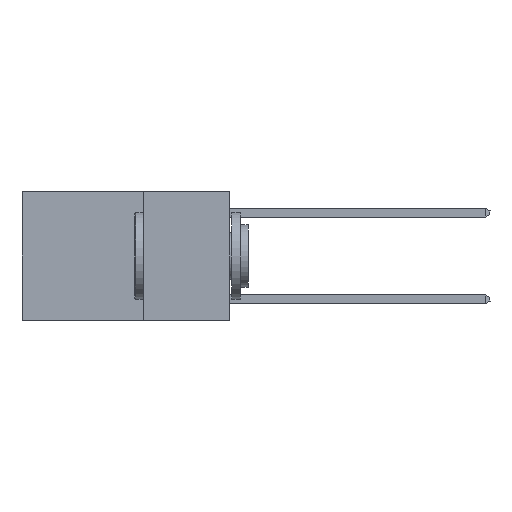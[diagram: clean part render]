
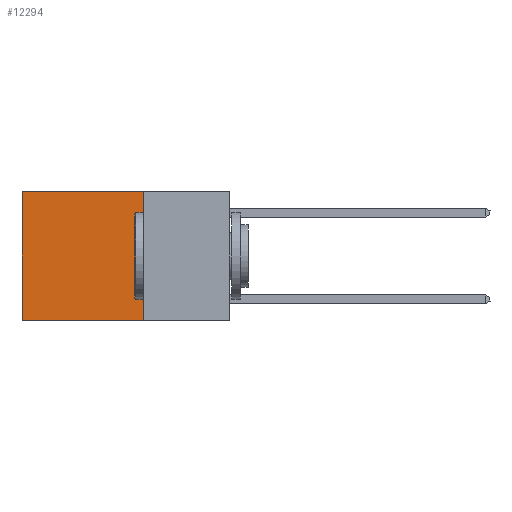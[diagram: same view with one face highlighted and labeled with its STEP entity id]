
A CAD part, left-side view. The second image highlights one B-rep face of the part: STEP entity #12294.
In plain terms, the highlighted planar face has unit normal (-1, 0, 0).
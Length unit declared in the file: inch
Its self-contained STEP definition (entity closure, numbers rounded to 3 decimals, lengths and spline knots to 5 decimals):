
#436 = EDGE_CURVE ( 'NONE', #13178, #13423, #4602, .T. ) ;
#2023 = PLANE ( 'NONE',  #14320 ) ;
#4602 = LINE ( 'NONE', #7304, #27635 ) ;
#5247 = CARTESIAN_POINT ( 'NONE',  ( 0.2625, 0.6, 0. ) ) ;
#5970 = ORIENTED_EDGE ( 'NONE', *, *, #11595, .T. ) ;
#6514 = DIRECTION ( 'NONE',  ( 0., 0., -1. ) ) ;
#6888 = CARTESIAN_POINT ( 'NONE',  ( 0.2625, 0.6, -0.37 ) ) ;
#7304 = CARTESIAN_POINT ( 'NONE',  ( 0.2625, 0.25, -0.37 ) ) ;
#7523 = CARTESIAN_POINT ( 'NONE',  ( 0.2625, 0.6, 0. ) ) ;
#7565 = VECTOR ( 'NONE', #11695, 39.37008 ) ;
#7737 = VERTEX_POINT ( 'NONE', #7523 ) ;
#9217 = DIRECTION ( 'NONE',  ( 1., 0., 0. ) ) ;
#9459 = CARTESIAN_POINT ( 'NONE',  ( 0.2625, 0.25, 0. ) ) ;
#9504 = EDGE_CURVE ( 'NONE', #7737, #13423, #11997, .T. ) ;
#11099 = CARTESIAN_POINT ( 'NONE',  ( 0.2625, 0.25, -0.37 ) ) ;
#11595 = EDGE_CURVE ( 'NONE', #11835, #7737, #28399, .T. ) ;
#11695 = DIRECTION ( 'NONE',  ( 0., 0., -1. ) ) ;
#11809 = VECTOR ( 'NONE', #27418, 39.37008 ) ;
#11835 = VERTEX_POINT ( 'NONE', #21680 ) ;
#11997 = LINE ( 'NONE', #5247, #11809 ) ;
#12188 = ORIENTED_EDGE ( 'NONE', *, *, #436, .F. ) ;
#12294 = ADVANCED_FACE ( 'NONE', ( #29546 ), #2023, .F. ) ;
#13178 = VERTEX_POINT ( 'NONE', #11099 ) ;
#13423 = VERTEX_POINT ( 'NONE', #6888 ) ;
#14320 = AXIS2_PLACEMENT_3D ( 'NONE', #24760, #9217, #6514 ) ;
#15012 = ORIENTED_EDGE ( 'NONE', *, *, #27944, .F. ) ;
#15457 = LINE ( 'NONE', #24570, #7565 ) ;
#16346 = DIRECTION ( 'NONE',  ( 0., 1., 0. ) ) ;
#21449 = EDGE_LOOP ( 'NONE', ( #21562, #12188, #15012, #5970 ) ) ;
#21562 = ORIENTED_EDGE ( 'NONE', *, *, #9504, .T. ) ;
#21680 = CARTESIAN_POINT ( 'NONE',  ( 0.2625, 0.25, 0. ) ) ;
#22860 = DIRECTION ( 'NONE',  ( 0., 1., 0. ) ) ;
#24570 = CARTESIAN_POINT ( 'NONE',  ( 0.2625, 0.25, 0. ) ) ;
#24760 = CARTESIAN_POINT ( 'NONE',  ( 0.2625, 0.25, 0. ) ) ;
#27418 = DIRECTION ( 'NONE',  ( 0., 0., -1. ) ) ;
#27635 = VECTOR ( 'NONE', #22860, 39.37008 ) ;
#27658 = VECTOR ( 'NONE', #16346, 39.37008 ) ;
#27944 = EDGE_CURVE ( 'NONE', #11835, #13178, #15457, .T. ) ;
#28399 = LINE ( 'NONE', #9459, #27658 ) ;
#29546 = FACE_OUTER_BOUND ( 'NONE', #21449, .T. ) ;
